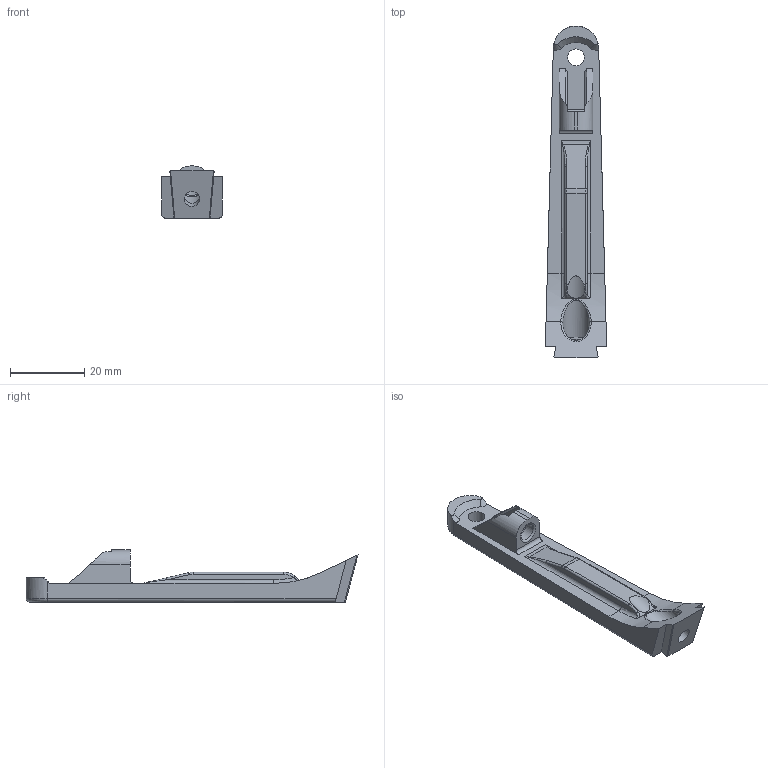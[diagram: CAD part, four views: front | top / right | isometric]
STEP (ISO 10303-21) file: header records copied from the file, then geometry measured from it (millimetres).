
FILE_DESCRIPTION(/* description */ (''),/* implementation_level */ '2;1');
FILE_NAME(/* name */ 'P.L.A. Tang.step',/* time_stamp */ '2022-06-19T00:29:26-05:00',/* author */ (''),/* organization */ (''),/* preprocessor_version */ 'ST-DEVELOPER v19',/* originating_system */ 'Autodesk Translation Framework v11.7.0.108',/* authorisation */ '');
FILE_SCHEMA (('AUTOMOTIVE_DESIGN { 1 0 10303 214 3 1 1 }'));
Length unit declared in the file: millimetre
Products named in the file (1): P.L.A. Tang
Bounding box: 16.47 x 89.25 x 14 mm (x, y, z)
Volume: 7565.6 mm3; surface area: 4391.7 mm2
Topology: 1 solids, 1 shells, 77 faces, 207 edges, 130 vertices
Faces by surface type: plane 33, cylinder 21, bspline 9, torus 9, cone 5
Full cylindrical faces by diameter (mm): 4.15 x1, 4.5 x1, 4.8 x1
Entity records: 2919 total; most frequent: CARTESIAN_POINT 979, ORIENTED_EDGE 410, DIRECTION 392, EDGE_CURVE 205, AXIS2_PLACEMENT_3D 145, VERTEX_POINT 130, LINE 102, VECTOR 102
